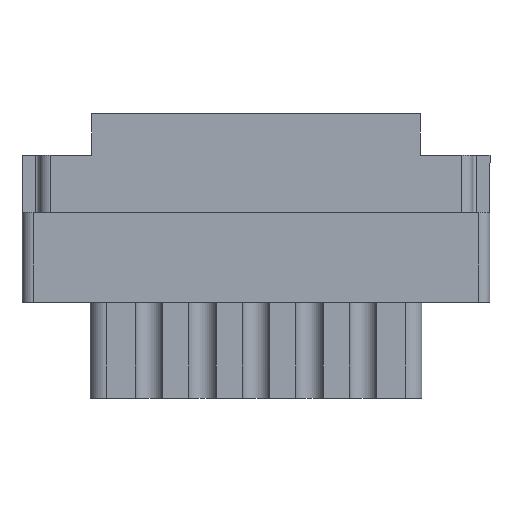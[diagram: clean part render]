
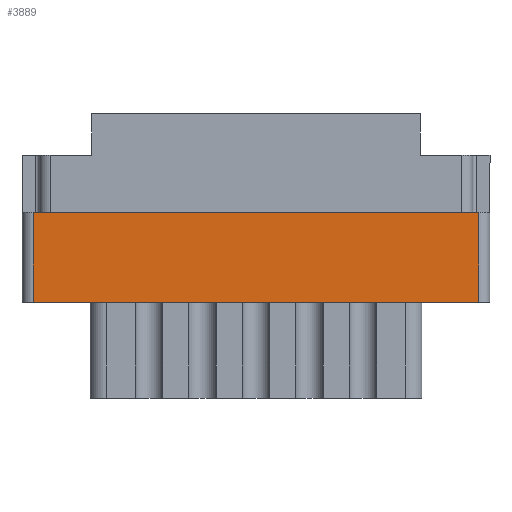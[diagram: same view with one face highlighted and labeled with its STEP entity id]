
A CAD part, front view. The second image highlights one B-rep face of the part: STEP entity #3889.
In plain terms, the highlighted planar face has unit normal (0, -1, 0).
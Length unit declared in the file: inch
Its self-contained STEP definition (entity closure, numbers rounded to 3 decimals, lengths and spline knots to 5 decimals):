
#183 = EDGE_CURVE ( 'NONE', #8421, #2570, #3241, .T. ) ;
#388 = DIRECTION ( 'NONE',  ( 0., -1., 0. ) ) ;
#734 = VECTOR ( 'NONE', #14516, 39.37008 ) ;
#758 = EDGE_CURVE ( 'NONE', #2570, #6531, #3040, .T. ) ;
#937 = CARTESIAN_POINT ( 'NONE',  ( -0.656, -0.343, -0.277 ) ) ;
#945 = EDGE_CURVE ( 'NONE', #8421, #4628, #9754, .T. ) ;
#1538 = CARTESIAN_POINT ( 'NONE',  ( -0.624, -0.343, -0.798 ) ) ;
#2570 = VERTEX_POINT ( 'NONE', #9437 ) ;
#2840 = ORIENTED_EDGE ( 'NONE', *, *, #4676, .F. ) ;
#2919 = DIRECTION ( 'NONE',  ( 0., 0., -1. ) ) ;
#3040 = LINE ( 'NONE', #7750, #9166 ) ;
#3241 = LINE ( 'NONE', #8186, #11282 ) ;
#3889 = ADVANCED_FACE ( 'NONE', ( #15187 ), #12751, .T. ) ;
#3947 = ORIENTED_EDGE ( 'NONE', *, *, #945, .T. ) ;
#4026 = ORIENTED_EDGE ( 'NONE', *, *, #758, .F. ) ;
#4628 = VERTEX_POINT ( 'NONE', #9792 ) ;
#4676 = EDGE_CURVE ( 'NONE', #6531, #4628, #11082, .T. ) ;
#5343 = CARTESIAN_POINT ( 'NONE',  ( 0.624, -0.343, -0.529 ) ) ;
#6531 = VERTEX_POINT ( 'NONE', #9365 ) ;
#7010 = CARTESIAN_POINT ( 'NONE',  ( 0.624, -0.343, -0.798 ) ) ;
#7750 = CARTESIAN_POINT ( 'NONE',  ( -0.624, -0.343, -0.798 ) ) ;
#8186 = CARTESIAN_POINT ( 'NONE',  ( 0.624, -0.343, -0.529 ) ) ;
#8358 = VECTOR ( 'NONE', #13110, 39.37008 ) ;
#8421 = VERTEX_POINT ( 'NONE', #5343 ) ;
#9166 = VECTOR ( 'NONE', #12714, 39.37008 ) ;
#9365 = CARTESIAN_POINT ( 'NONE',  ( -0.624, -0.343, -0.277 ) ) ;
#9437 = CARTESIAN_POINT ( 'NONE',  ( -0.624, -0.343, -0.529 ) ) ;
#9754 = LINE ( 'NONE', #7010, #8358 ) ;
#9792 = CARTESIAN_POINT ( 'NONE',  ( 0.624, -0.343, -0.277 ) ) ;
#9927 = ORIENTED_EDGE ( 'NONE', *, *, #183, .F. ) ;
#10397 = EDGE_LOOP ( 'NONE', ( #4026, #9927, #3947, #2840 ) ) ;
#11082 = LINE ( 'NONE', #937, #734 ) ;
#11282 = VECTOR ( 'NONE', #13152, 39.37008 ) ;
#12714 = DIRECTION ( 'NONE',  ( 0., 0., 1. ) ) ;
#12751 = PLANE ( 'NONE',  #15771 ) ;
#13110 = DIRECTION ( 'NONE',  ( 0., 0., 1. ) ) ;
#13152 = DIRECTION ( 'NONE',  ( -1., 0., 0. ) ) ;
#14516 = DIRECTION ( 'NONE',  ( 1., 0., 0. ) ) ;
#15187 = FACE_OUTER_BOUND ( 'NONE', #10397, .T. ) ;
#15771 = AXIS2_PLACEMENT_3D ( 'NONE', #1538, #388, #2919 ) ;
